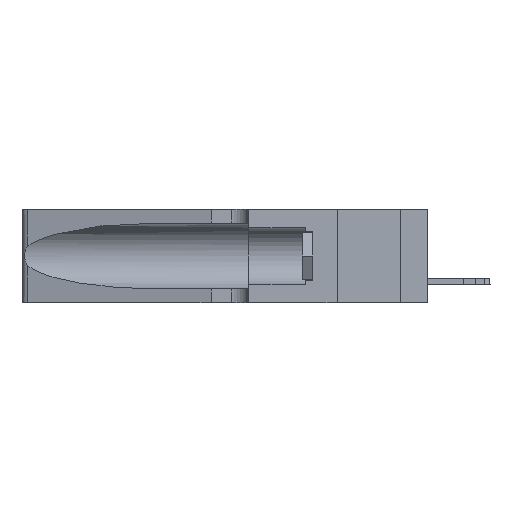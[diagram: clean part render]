
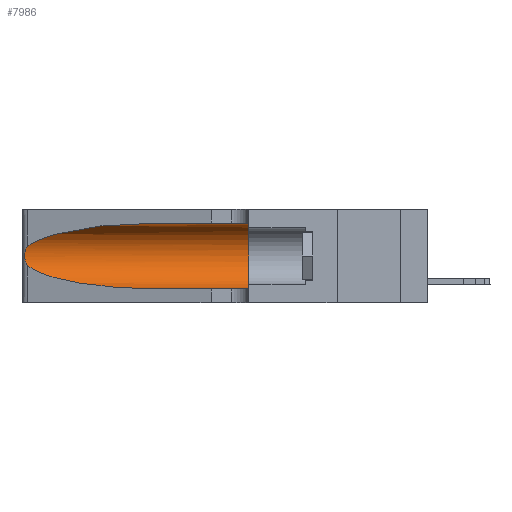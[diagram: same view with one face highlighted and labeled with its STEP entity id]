
A CAD part, left-side view. The second image highlights one B-rep face of the part: STEP entity #7986.
In plain terms, the highlighted cylindrical face has radius 3.308 mm (diameter 6.617 mm), a partial arc.
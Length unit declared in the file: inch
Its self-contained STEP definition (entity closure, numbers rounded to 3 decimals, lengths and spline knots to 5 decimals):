
#232 = CARTESIAN_POINT ( 'NONE',  ( 0.25487, 1.22718, 0.14631 ) ) ;
#608 = VECTOR ( 'NONE', #8011, 39.37008 ) ;
#1025 = CARTESIAN_POINT ( 'NONE',  ( 0.2373, 1.15595, 0.28018 ) ) ;
#1276 = CARTESIAN_POINT ( 'NONE',  ( 0.25639, 1.23186, 0.15144 ) ) ;
#2447 = CARTESIAN_POINT ( 'NONE',  ( 0.18966, 0.96281, 0.05475 ) ) ;
#2922 = CARTESIAN_POINT ( 'NONE',  ( 0.25787, 1.23484, 0.2124 ) ) ;
#3921 =( BOUNDED_CURVE ( )  B_SPLINE_CURVE ( 3, ( #32477, #17261, #2447, #32140 ),
 .UNSPECIFIED., .F., .T. ) 
 B_SPLINE_CURVE_WITH_KNOTS ( ( 4, 4 ),
 ( 3.44316, 4.71239 ),
 .UNSPECIFIED. ) 
 CURVE ( )  GEOMETRIC_REPRESENTATION_ITEM ( )  RATIONAL_B_SPLINE_CURVE ( ( 1., 0.87, 0.87, 1. ) ) 
 REPRESENTATION_ITEM ( '' )  );
#4156 = LINE ( 'NONE', #5477, #608 ) ;
#4284 = EDGE_CURVE ( 'NONE', #18083, #4743, #29669, .T. ) ;
#4576 = ORIENTED_EDGE ( 'NONE', *, *, #8037, .T. ) ;
#4743 = VERTEX_POINT ( 'NONE', #232 ) ;
#4920 = DIRECTION ( 'NONE',  ( 0., 0., 1. ) ) ;
#5477 = CARTESIAN_POINT ( 'NONE',  ( 0.1305, 1.61858, 0.31525 ) ) ;
#6630 = ORIENTED_EDGE ( 'NONE', *, *, #24489, .F. ) ;
#7296 = EDGE_CURVE ( 'NONE', #20376, #27855, #23976, .T. ) ;
#7864 = CARTESIAN_POINT ( 'NONE',  ( 0.25555, 1.22994, 0.2215 ) ) ;
#7969 = CARTESIAN_POINT ( 'NONE',  ( 0.25854, 1.2359, 0.20912 ) ) ;
#7986 = ADVANCED_FACE ( 'NONE', ( #14997 ), #25288, .F. ) ;
#8011 = DIRECTION ( 'NONE',  ( 0., -1., 0. ) ) ;
#8037 = EDGE_CURVE ( 'NONE', #31883, #18083, #21447, .T. ) ;
#8617 = CARTESIAN_POINT ( 'NONE',  ( 0.1305, 0.72297, 0.31525 ) ) ;
#8638 = CARTESIAN_POINT ( 'NONE',  ( 0.25789, 1.23486, 0.15765 ) ) ;
#8723 = CARTESIAN_POINT ( 'NONE',  ( 0.1305, 0.72297, 0.05475 ) ) ;
#8954 = CARTESIAN_POINT ( 'NONE',  ( 0.25487, 1.22718, 0.14631 ) ) ;
#8958 = ORIENTED_EDGE ( 'NONE', *, *, #24823, .T. ) ;
#10395 = EDGE_LOOP ( 'NONE', ( #4576, #25093, #8958, #21259, #30645, #6630 ) ) ;
#12972 = CARTESIAN_POINT ( 'NONE',  ( 0.26018, 1.23835, 0.19895 ) ) ;
#13203 = CARTESIAN_POINT ( 'NONE',  ( 0.25487, 1.22718, 0.22369 ) ) ;
#14997 = FACE_OUTER_BOUND ( 'NONE', #10395, .T. ) ;
#15310 = CIRCLE ( 'NONE', #15710, 0.13025 ) ;
#15662 = AXIS2_PLACEMENT_3D ( 'NONE', #31428, #28544, #31104 ) ;
#15710 = AXIS2_PLACEMENT_3D ( 'NONE', #22205, #27451, #4920 ) ;
#15852 = CARTESIAN_POINT ( 'NONE',  ( 0.1305, 0.72297, 0.31525 ) ) ;
#16043 = CARTESIAN_POINT ( 'NONE',  ( 0.25487, 1.22718, 0.22369 ) ) ;
#16276 = CARTESIAN_POINT ( 'NONE',  ( 0.26017, 1.23833, 0.17102 ) ) ;
#16305 = CARTESIAN_POINT ( 'NONE',  ( 0.18966, 0.96281, 0.31525 ) ) ;
#17261 = CARTESIAN_POINT ( 'NONE',  ( 0.2373, 1.15595, 0.08982 ) ) ;
#18083 = VERTEX_POINT ( 'NONE', #16043 ) ;
#18440 = CARTESIAN_POINT ( 'NONE',  ( 0.1305, 0.35, 0.31525 ) ) ;
#18628 = CARTESIAN_POINT ( 'NONE',  ( 0.25856, 1.23593, 0.16098 ) ) ;
#18854 = VECTOR ( 'NONE', #19996, 39.37008 ) ;
#19996 = DIRECTION ( 'NONE',  ( 0., -1., 0. ) ) ;
#20376 = VERTEX_POINT ( 'NONE', #8723 ) ;
#20621 = CARTESIAN_POINT ( 'NONE',  ( 0.26075, 1.23896, 0.19203 ) ) ;
#21259 = ORIENTED_EDGE ( 'NONE', *, *, #7296, .T. ) ;
#21415 = CARTESIAN_POINT ( 'NONE',  ( 0.26075, 1.23896, 0.178 ) ) ;
#21447 =( BOUNDED_CURVE ( )  B_SPLINE_CURVE ( 3, ( #15852, #16305, #1025, #28994 ),
 .UNSPECIFIED., .F., .F. ) 
 B_SPLINE_CURVE_WITH_KNOTS ( ( 4, 4 ),
 ( 1.5708, 2.84003 ),
 .UNSPECIFIED. ) 
 CURVE ( )  GEOMETRIC_REPRESENTATION_ITEM ( )  RATIONAL_B_SPLINE_CURVE ( ( 1., 0.87, 0.87, 1. ) ) 
 REPRESENTATION_ITEM ( '' )  );
#22205 = CARTESIAN_POINT ( 'NONE',  ( 0.1305, 0.35, 0.185 ) ) ;
#22416 = CARTESIAN_POINT ( 'NONE',  ( 0.1305, 1.61858, 0.05475 ) ) ;
#23976 = LINE ( 'NONE', #22416, #18854 ) ;
#24489 = EDGE_CURVE ( 'NONE', #31883, #24636, #4156, .T. ) ;
#24636 = VERTEX_POINT ( 'NONE', #18440 ) ;
#24823 = EDGE_CURVE ( 'NONE', #4743, #20376, #3921, .T. ) ;
#25093 = ORIENTED_EDGE ( 'NONE', *, *, #4284, .T. ) ;
#25288 = CYLINDRICAL_SURFACE ( 'NONE', #15662, 0.13025 ) ;
#27451 = DIRECTION ( 'NONE',  ( 0., 1., 0. ) ) ;
#27855 = VERTEX_POINT ( 'NONE', #28821 ) ;
#28544 = DIRECTION ( 'NONE',  ( 0., -1., 0. ) ) ;
#28773 = EDGE_CURVE ( 'NONE', #24636, #27855, #15310, .T. ) ;
#28821 = CARTESIAN_POINT ( 'NONE',  ( 0.1305, 0.35, 0.05475 ) ) ;
#28994 = CARTESIAN_POINT ( 'NONE',  ( 0.25487, 1.22718, 0.22369 ) ) ;
#29669 = B_SPLINE_CURVE_WITH_KNOTS ( 'NONE', 3,
 ( #13203, #7864, #30498, #2922, #7969, #12972, #20621, #21415, #16276, #18628, #8638, #1276, #31829, #8954 ),
 .UNSPECIFIED., .F., .F.,
 ( 4, 2, 2, 2, 2, 2, 4 ),
 ( 0., 0.00027, 0.00053, 0.00107, 0.0016, 0.00187, 0.00214 ),
 .UNSPECIFIED. ) ;
#30498 = CARTESIAN_POINT ( 'NONE',  ( 0.25639, 1.23184, 0.21858 ) ) ;
#30645 = ORIENTED_EDGE ( 'NONE', *, *, #28773, .F. ) ;
#31104 = DIRECTION ( 'NONE',  ( 0., 0., -1. ) ) ;
#31428 = CARTESIAN_POINT ( 'NONE',  ( 0.1305, 1.61858, 0.185 ) ) ;
#31829 = CARTESIAN_POINT ( 'NONE',  ( 0.25555, 1.22993, 0.14849 ) ) ;
#31883 = VERTEX_POINT ( 'NONE', #8617 ) ;
#32140 = CARTESIAN_POINT ( 'NONE',  ( 0.1305, 0.72297, 0.05475 ) ) ;
#32477 = CARTESIAN_POINT ( 'NONE',  ( 0.25487, 1.22718, 0.14631 ) ) ;
